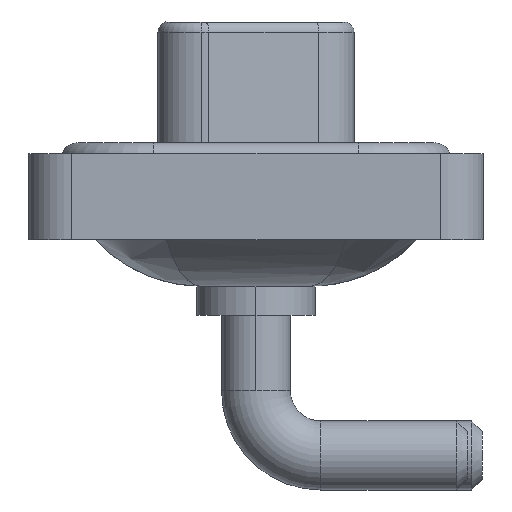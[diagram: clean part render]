
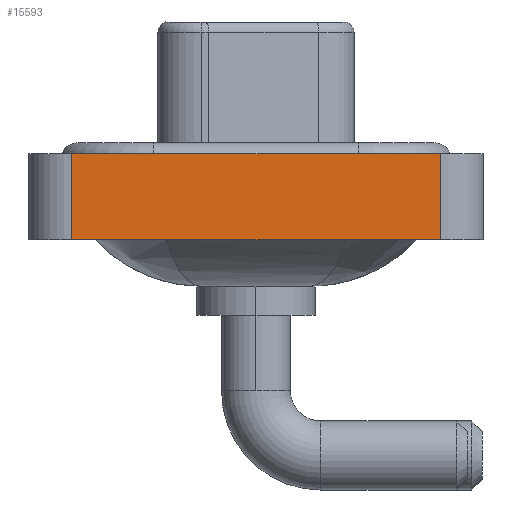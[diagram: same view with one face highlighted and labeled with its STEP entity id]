
A CAD part, left-side view. The second image highlights one B-rep face of the part: STEP entity #15593.
In plain terms, the highlighted planar face has unit normal (-1, 0, 0).
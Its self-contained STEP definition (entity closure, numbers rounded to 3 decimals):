
#211 = ORIENTED_EDGE ( 'NONE', *, *, #4988, .F. ) ;
#866 = ORIENTED_EDGE ( 'NONE', *, *, #14306, .T. ) ;
#2088 = VERTEX_POINT ( 'NONE', #3447 ) ;
#2420 = CARTESIAN_POINT ( 'NONE',  ( -7.3, -8.55, -3.6 ) ) ;
#2712 = DIRECTION ( 'NONE',  ( 0., 0., 1. ) ) ;
#2719 = CARTESIAN_POINT ( 'NONE',  ( -7.3, -8.55, 0.4 ) ) ;
#3220 = VECTOR ( 'NONE', #10320, 1000. ) ;
#3447 = CARTESIAN_POINT ( 'NONE',  ( -7.3, 8.55, -3.6 ) ) ;
#3958 = LINE ( 'NONE', #2420, #13391 ) ;
#4060 = LINE ( 'NONE', #2719, #3220 ) ;
#4249 = CARTESIAN_POINT ( 'NONE',  ( -7.3, -8.55, -3.6 ) ) ;
#4988 = EDGE_CURVE ( 'NONE', #14179, #5511, #4060, .T. ) ;
#5412 = DIRECTION ( 'NONE',  ( 0., -1., 0. ) ) ;
#5511 = VERTEX_POINT ( 'NONE', #6050 ) ;
#5684 = DIRECTION ( 'NONE',  ( 0., 0., 1. ) ) ;
#5930 = VECTOR ( 'NONE', #5412, 1000. ) ;
#6050 = CARTESIAN_POINT ( 'NONE',  ( -7.3, -8.55, 0.4 ) ) ;
#6870 = DIRECTION ( 'NONE',  ( 0., 0., 1. ) ) ;
#6974 = LINE ( 'NONE', #4249, #5930 ) ;
#7283 = CARTESIAN_POINT ( 'NONE',  ( -7.3, -8.55, -3.6 ) ) ;
#8255 = ORIENTED_EDGE ( 'NONE', *, *, #18784, .T. ) ;
#8735 = FACE_OUTER_BOUND ( 'NONE', #11999, .T. ) ;
#9634 = VECTOR ( 'NONE', #5684, 1000. ) ;
#9724 = CARTESIAN_POINT ( 'NONE',  ( -7.3, 8.55, 0.4 ) ) ;
#9925 = PLANE ( 'NONE',  #17515 ) ;
#10320 = DIRECTION ( 'NONE',  ( 0., -1., 0. ) ) ;
#11999 = EDGE_LOOP ( 'NONE', ( #8255, #211, #14580, #866 ) ) ;
#13391 = VECTOR ( 'NONE', #6870, 1000. ) ;
#14118 = VERTEX_POINT ( 'NONE', #18396 ) ;
#14179 = VERTEX_POINT ( 'NONE', #9724 ) ;
#14198 = CARTESIAN_POINT ( 'NONE',  ( -7.3, 8.55, -3.6 ) ) ;
#14306 = EDGE_CURVE ( 'NONE', #2088, #14118, #6974, .T. ) ;
#14580 = ORIENTED_EDGE ( 'NONE', *, *, #19133, .F. ) ;
#15593 = ADVANCED_FACE ( 'NONE', ( #8735 ), #9925, .T. ) ;
#15669 = LINE ( 'NONE', #14198, #9634 ) ;
#17515 = AXIS2_PLACEMENT_3D ( 'NONE', #7283, #17541, #2712 ) ;
#17541 = DIRECTION ( 'NONE',  ( -1., 0., 0. ) ) ;
#18396 = CARTESIAN_POINT ( 'NONE',  ( -7.3, -8.55, -3.6 ) ) ;
#18784 = EDGE_CURVE ( 'NONE', #14118, #5511, #3958, .T. ) ;
#19133 = EDGE_CURVE ( 'NONE', #2088, #14179, #15669, .T. ) ;
